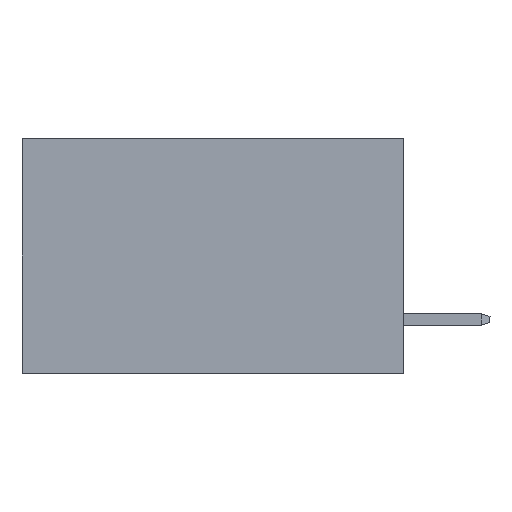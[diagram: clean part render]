
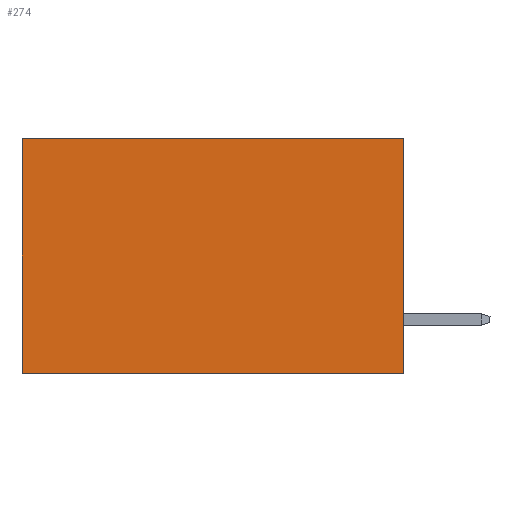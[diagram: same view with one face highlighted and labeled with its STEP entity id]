
A CAD part, left-side view. The second image highlights one B-rep face of the part: STEP entity #274.
In plain terms, the highlighted planar face has unit normal (-1, 0, 0).
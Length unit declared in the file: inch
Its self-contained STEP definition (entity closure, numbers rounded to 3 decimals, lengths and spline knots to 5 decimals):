
#46 = CARTESIAN_POINT ( 'NONE',  ( 0.2875, 0., -0.37 ) ) ;
#75 = DIRECTION ( 'NONE',  ( 0., 0., -1. ) ) ;
#274 = ADVANCED_FACE ( 'NONE', ( #889 ), #1492, .F. ) ;
#509 = VECTOR ( 'NONE', #7126, 39.37008 ) ;
#770 = CARTESIAN_POINT ( 'NONE',  ( 0.2875, 0.6, 0. ) ) ;
#889 = FACE_OUTER_BOUND ( 'NONE', #7796, .T. ) ;
#1179 = CARTESIAN_POINT ( 'NONE',  ( 0.2875, 0., 0. ) ) ;
#1404 = DIRECTION ( 'NONE',  ( 1., 0., 0. ) ) ;
#1492 = PLANE ( 'NONE',  #7437 ) ;
#1613 = VERTEX_POINT ( 'NONE', #7732 ) ;
#1638 = CARTESIAN_POINT ( 'NONE',  ( 0.2875, 0., -0.37 ) ) ;
#1739 = ORIENTED_EDGE ( 'NONE', *, *, #2408, .T. ) ;
#2408 = EDGE_CURVE ( 'NONE', #7824, #6017, #6740, .T. ) ;
#2679 = ORIENTED_EDGE ( 'NONE', *, *, #3459, .T. ) ;
#2958 = VERTEX_POINT ( 'NONE', #1638 ) ;
#3459 = EDGE_CURVE ( 'NONE', #1613, #7824, #4464, .T. ) ;
#3514 = EDGE_CURVE ( 'NONE', #2958, #6017, #6515, .T. ) ;
#3518 = CARTESIAN_POINT ( 'NONE',  ( 0.2875, 0., 0. ) ) ;
#4231 = VECTOR ( 'NONE', #7082, 39.37008 ) ;
#4239 = VECTOR ( 'NONE', #4751, 39.37008 ) ;
#4275 = VECTOR ( 'NONE', #75, 39.37008 ) ;
#4436 = ORIENTED_EDGE ( 'NONE', *, *, #3514, .F. ) ;
#4464 = LINE ( 'NONE', #1179, #4231 ) ;
#4738 = DIRECTION ( 'NONE',  ( 0., 0., -1. ) ) ;
#4751 = DIRECTION ( 'NONE',  ( 0., 0., -1. ) ) ;
#5162 = ORIENTED_EDGE ( 'NONE', *, *, #7607, .F. ) ;
#5476 = CARTESIAN_POINT ( 'NONE',  ( 0.2875, 0., 0. ) ) ;
#5779 = CARTESIAN_POINT ( 'NONE',  ( 0.2875, 0.6, 0. ) ) ;
#5969 = LINE ( 'NONE', #5476, #4275 ) ;
#6017 = VERTEX_POINT ( 'NONE', #7768 ) ;
#6515 = LINE ( 'NONE', #46, #509 ) ;
#6740 = LINE ( 'NONE', #770, #4239 ) ;
#7082 = DIRECTION ( 'NONE',  ( 0., 1., 0. ) ) ;
#7126 = DIRECTION ( 'NONE',  ( 0., 1., 0. ) ) ;
#7437 = AXIS2_PLACEMENT_3D ( 'NONE', #3518, #1404, #4738 ) ;
#7607 = EDGE_CURVE ( 'NONE', #1613, #2958, #5969, .T. ) ;
#7732 = CARTESIAN_POINT ( 'NONE',  ( 0.2875, 0., 0. ) ) ;
#7768 = CARTESIAN_POINT ( 'NONE',  ( 0.2875, 0.6, -0.37 ) ) ;
#7796 = EDGE_LOOP ( 'NONE', ( #1739, #4436, #5162, #2679 ) ) ;
#7824 = VERTEX_POINT ( 'NONE', #5779 ) ;
